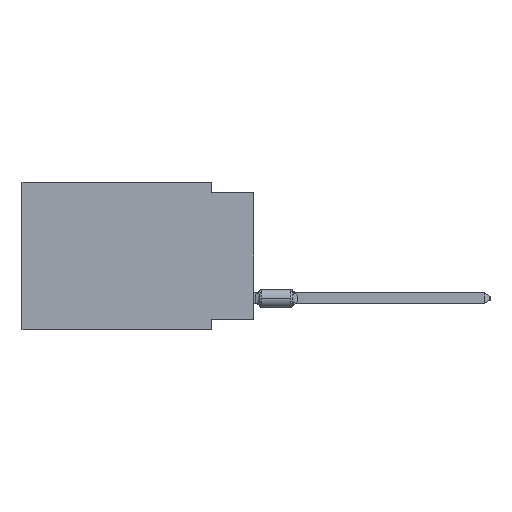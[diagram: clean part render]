
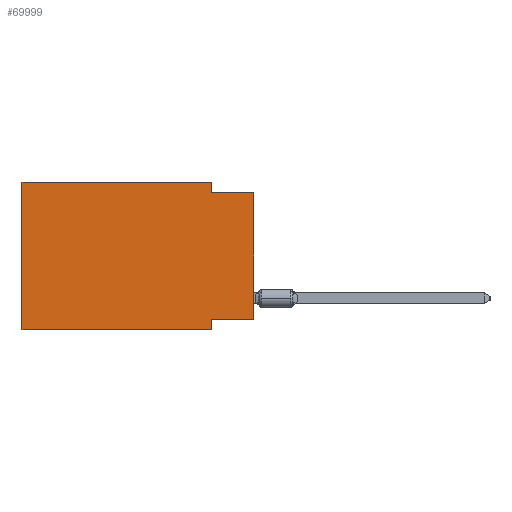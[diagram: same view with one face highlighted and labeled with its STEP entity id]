
A CAD part, left-side view. The second image highlights one B-rep face of the part: STEP entity #69999.
In plain terms, the highlighted planar face has unit normal (-1, 0, 0).
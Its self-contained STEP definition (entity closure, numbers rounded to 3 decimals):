
#1584 = VECTOR ( 'NONE', #4256, 1000. ) ;
#4256 = DIRECTION ( 'NONE',  ( 0., 0., -1. ) ) ;
#5570 = CARTESIAN_POINT ( 'NONE',  ( 0., 13.97, -8.89 ) ) ;
#5615 = DIRECTION ( 'NONE',  ( 0., -1., 0. ) ) ;
#11996 = CARTESIAN_POINT ( 'NONE',  ( 0., 13.97, 0. ) ) ;
#12389 = LINE ( 'NONE', #78517, #1584 ) ;
#15110 = CARTESIAN_POINT ( 'NONE',  ( 0., 0., 0. ) ) ;
#15606 = EDGE_CURVE ( 'NONE', #58890, #88189, #70489, .T. ) ;
#19043 = CARTESIAN_POINT ( 'NONE',  ( 0., 13.97, 0. ) ) ;
#20107 = VECTOR ( 'NONE', #51024, 1000. ) ;
#20653 = DIRECTION ( 'NONE',  ( 0., 0., -1. ) ) ;
#21228 = DIRECTION ( 'NONE',  ( 0., 1., 0. ) ) ;
#23562 = ORIENTED_EDGE ( 'NONE', *, *, #25595, .F. ) ;
#25595 = EDGE_CURVE ( 'NONE', #42588, #58890, #59698, .T. ) ;
#26051 = VECTOR ( 'NONE', #86892, 1000. ) ;
#29710 = ORIENTED_EDGE ( 'NONE', *, *, #46232, .F. ) ;
#34589 = CARTESIAN_POINT ( 'NONE',  ( 0., 2.54, -0.635 ) ) ;
#34800 = VECTOR ( 'NONE', #5615, 1000. ) ;
#36163 = CARTESIAN_POINT ( 'NONE',  ( 0., 2.54, -8.255 ) ) ;
#38837 = ORIENTED_EDGE ( 'NONE', *, *, #41177, .T. ) ;
#39720 = ORIENTED_EDGE ( 'NONE', *, *, #39905, .F. ) ;
#39905 = EDGE_CURVE ( 'NONE', #57217, #42032, #12389, .T. ) ;
#39946 = VERTEX_POINT ( 'NONE', #56865 ) ;
#41177 = EDGE_CURVE ( 'NONE', #42588, #42032, #79289, .T. ) ;
#42032 = VERTEX_POINT ( 'NONE', #106303 ) ;
#42588 = VERTEX_POINT ( 'NONE', #51929 ) ;
#45219 = CARTESIAN_POINT ( 'NONE',  ( 0., 0., -0.635 ) ) ;
#45566 = VECTOR ( 'NONE', #79632, 1000. ) ;
#46232 = EDGE_CURVE ( 'NONE', #88189, #101173, #68445, .T. ) ;
#46566 = LINE ( 'NONE', #15110, #45566 ) ;
#48383 = VECTOR ( 'NONE', #69956, 1000. ) ;
#49885 = ORIENTED_EDGE ( 'NONE', *, *, #66349, .F. ) ;
#51024 = DIRECTION ( 'NONE',  ( 0., 0., 1. ) ) ;
#51280 = ORIENTED_EDGE ( 'NONE', *, *, #92499, .F. ) ;
#51929 = CARTESIAN_POINT ( 'NONE',  ( 0., 13.97, -8.89 ) ) ;
#53201 = LINE ( 'NONE', #53752, #63027 ) ;
#53752 = CARTESIAN_POINT ( 'NONE',  ( 0., 0., -8.255 ) ) ;
#54283 = EDGE_CURVE ( 'NONE', #39946, #56431, #46566, .T. ) ;
#56431 = VERTEX_POINT ( 'NONE', #69094 ) ;
#56865 = CARTESIAN_POINT ( 'NONE',  ( 0., 0., -8.255 ) ) ;
#57217 = VERTEX_POINT ( 'NONE', #36163 ) ;
#58890 = VERTEX_POINT ( 'NONE', #88569 ) ;
#59698 = LINE ( 'NONE', #92737, #20107 ) ;
#60787 = DIRECTION ( 'NONE',  ( 1., 0., 0. ) ) ;
#61630 = ORIENTED_EDGE ( 'NONE', *, *, #54283, .T. ) ;
#63027 = VECTOR ( 'NONE', #21228, 1000. ) ;
#66349 = EDGE_CURVE ( 'NONE', #101173, #56431, #79335, .T. ) ;
#68445 = LINE ( 'NONE', #77666, #106166 ) ;
#69094 = CARTESIAN_POINT ( 'NONE',  ( 0., 0., -0.635 ) ) ;
#69449 = FACE_OUTER_BOUND ( 'NONE', #100950, .T. ) ;
#69956 = DIRECTION ( 'NONE',  ( 0., -1., 0. ) ) ;
#69999 = ADVANCED_FACE ( 'NONE', ( #69449 ), #85705, .F. ) ;
#70489 = LINE ( 'NONE', #19043, #48383 ) ;
#73694 = CARTESIAN_POINT ( 'NONE',  ( 0., 2.54, 0. ) ) ;
#77666 = CARTESIAN_POINT ( 'NONE',  ( 0., 2.54, 0. ) ) ;
#78517 = CARTESIAN_POINT ( 'NONE',  ( 0., 2.54, -8.89 ) ) ;
#79289 = LINE ( 'NONE', #5570, #26051 ) ;
#79335 = LINE ( 'NONE', #45219, #34800 ) ;
#79632 = DIRECTION ( 'NONE',  ( 0., 0., 1. ) ) ;
#83667 = DIRECTION ( 'NONE',  ( 0., 0., -1. ) ) ;
#85320 = AXIS2_PLACEMENT_3D ( 'NONE', #11996, #60787, #20653 ) ;
#85705 = PLANE ( 'NONE',  #85320 ) ;
#86892 = DIRECTION ( 'NONE',  ( 0., -1., 0. ) ) ;
#88189 = VERTEX_POINT ( 'NONE', #73694 ) ;
#88569 = CARTESIAN_POINT ( 'NONE',  ( 0., 13.97, 0. ) ) ;
#92499 = EDGE_CURVE ( 'NONE', #39946, #57217, #53201, .T. ) ;
#92737 = CARTESIAN_POINT ( 'NONE',  ( 0., 13.97, 0. ) ) ;
#95332 = ORIENTED_EDGE ( 'NONE', *, *, #15606, .F. ) ;
#100950 = EDGE_LOOP ( 'NONE', ( #61630, #49885, #29710, #95332, #23562, #38837, #39720, #51280 ) ) ;
#101173 = VERTEX_POINT ( 'NONE', #34589 ) ;
#106166 = VECTOR ( 'NONE', #83667, 1000. ) ;
#106303 = CARTESIAN_POINT ( 'NONE',  ( 0., 2.54, -8.89 ) ) ;
